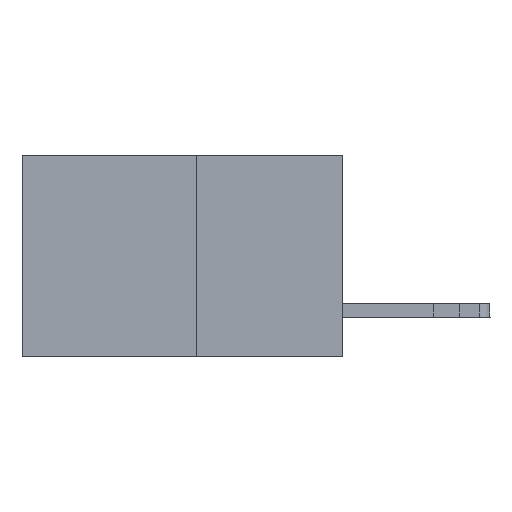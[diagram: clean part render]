
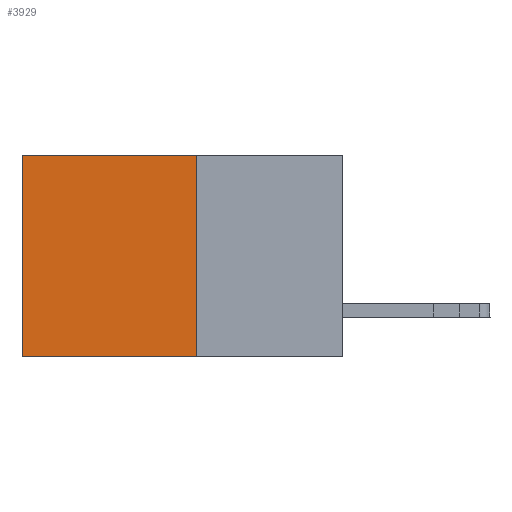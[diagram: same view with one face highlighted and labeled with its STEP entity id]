
A CAD part, left-side view. The second image highlights one B-rep face of the part: STEP entity #3929.
In plain terms, the highlighted planar face has unit normal (-1, 0, 0).
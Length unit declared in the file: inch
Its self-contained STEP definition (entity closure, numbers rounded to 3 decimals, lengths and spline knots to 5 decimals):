
#481 = ORIENTED_EDGE ( 'NONE', *, *, #21215, .T. ) ;
#656 = DIRECTION ( 'NONE',  ( 0., 1., 0. ) ) ;
#1170 = FACE_OUTER_BOUND ( 'NONE', #7653, .T. ) ;
#1537 = VECTOR ( 'NONE', #7393, 39.37008 ) ;
#2607 = LINE ( 'NONE', #23688, #1537 ) ;
#2666 = CARTESIAN_POINT ( 'NONE',  ( 0.277, 0.27, -0.37 ) ) ;
#3929 = ADVANCED_FACE ( 'NONE', ( #1170 ), #17833, .F. ) ;
#5135 = ORIENTED_EDGE ( 'NONE', *, *, #9291, .T. ) ;
#5240 = LINE ( 'NONE', #13443, #8356 ) ;
#7261 = CARTESIAN_POINT ( 'NONE',  ( 0.277, 0.27, -0.37 ) ) ;
#7393 = DIRECTION ( 'NONE',  ( 0., 0., -1. ) ) ;
#7473 = CARTESIAN_POINT ( 'NONE',  ( 0.277, 0.27, -0.37 ) ) ;
#7653 = EDGE_LOOP ( 'NONE', ( #481, #10497, #9311, #5135 ) ) ;
#7882 = VERTEX_POINT ( 'NONE', #7261 ) ;
#8356 = VECTOR ( 'NONE', #21661, 39.37008 ) ;
#9291 = EDGE_CURVE ( 'NONE', #17598, #12617, #5240, .T. ) ;
#9311 = ORIENTED_EDGE ( 'NONE', *, *, #21544, .F. ) ;
#10143 = VECTOR ( 'NONE', #656, 39.37008 ) ;
#10497 = ORIENTED_EDGE ( 'NONE', *, *, #21888, .F. ) ;
#10767 = CARTESIAN_POINT ( 'NONE',  ( 0.277, 0.59, -0.37 ) ) ;
#12617 = VERTEX_POINT ( 'NONE', #22786 ) ;
#13443 = CARTESIAN_POINT ( 'NONE',  ( 0.277, 0.27, 0. ) ) ;
#14960 = CARTESIAN_POINT ( 'NONE',  ( 0.277, 0.27, 0. ) ) ;
#17598 = VERTEX_POINT ( 'NONE', #14960 ) ;
#17833 = PLANE ( 'NONE',  #21186 ) ;
#19355 = LINE ( 'NONE', #2666, #10143 ) ;
#19605 = DIRECTION ( 'NONE',  ( 1., 0., 0. ) ) ;
#20049 = CARTESIAN_POINT ( 'NONE',  ( 0.277, 0.59, -0.37 ) ) ;
#21186 = AXIS2_PLACEMENT_3D ( 'NONE', #7473, #19605, #21886 ) ;
#21215 = EDGE_CURVE ( 'NONE', #12617, #24703, #23817, .T. ) ;
#21544 = EDGE_CURVE ( 'NONE', #17598, #7882, #2607, .T. ) ;
#21661 = DIRECTION ( 'NONE',  ( 0., 1., 0. ) ) ;
#21886 = DIRECTION ( 'NONE',  ( 0., 0., -1. ) ) ;
#21888 = EDGE_CURVE ( 'NONE', #7882, #24703, #19355, .T. ) ;
#22786 = CARTESIAN_POINT ( 'NONE',  ( 0.277, 0.59, 0. ) ) ;
#23688 = CARTESIAN_POINT ( 'NONE',  ( 0.277, 0.27, -0.37 ) ) ;
#23817 = LINE ( 'NONE', #20049, #26450 ) ;
#24703 = VERTEX_POINT ( 'NONE', #10767 ) ;
#25710 = DIRECTION ( 'NONE',  ( 0., 0., -1. ) ) ;
#26450 = VECTOR ( 'NONE', #25710, 39.37008 ) ;
